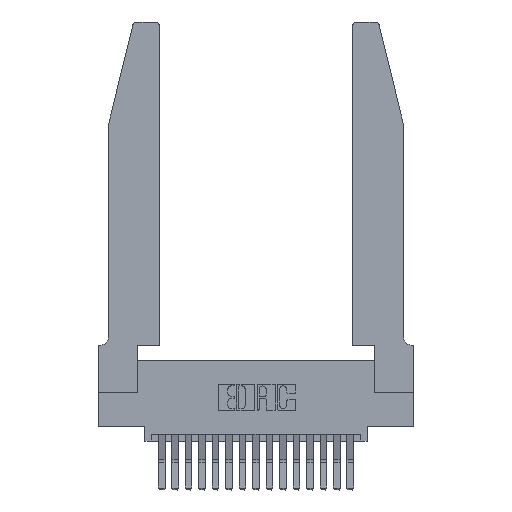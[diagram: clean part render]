
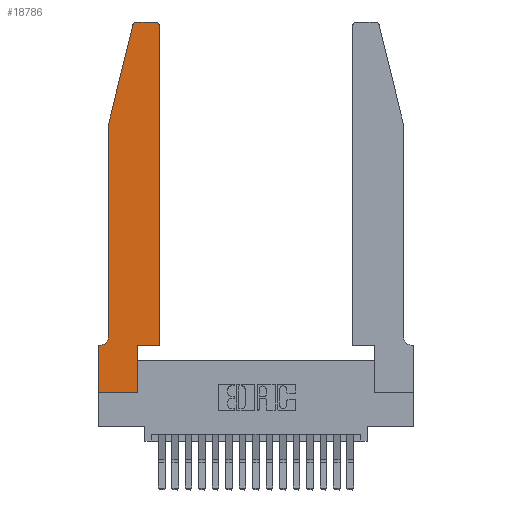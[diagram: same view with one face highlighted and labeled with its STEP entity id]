
A CAD part, top view. The second image highlights one B-rep face of the part: STEP entity #18786.
In plain terms, the highlighted planar face has unit normal (0, 0, 1).
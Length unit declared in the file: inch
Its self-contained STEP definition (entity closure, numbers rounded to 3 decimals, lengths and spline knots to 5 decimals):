
#42 = CARTESIAN_POINT ( 'NONE',  ( 0.2865, 0., 0.37 ) ) ;
#189 = DIRECTION ( 'NONE',  ( 0., -1., 0. ) ) ;
#421 = EDGE_CURVE ( 'NONE', #17162, #8743, #11018, .T. ) ;
#666 = DIRECTION ( 'NONE',  ( -1., 0., 0. ) ) ;
#910 = VERTEX_POINT ( 'NONE', #7275 ) ;
#926 = CARTESIAN_POINT ( 'NONE',  ( 0.4205, 2.75, 0.37 ) ) ;
#972 = FACE_OUTER_BOUND ( 'NONE', #2865, .T. ) ;
#1042 = ORIENTED_EDGE ( 'NONE', *, *, #15183, .T. ) ;
#1206 = VECTOR ( 'NONE', #11545, 39.37008 ) ;
#1276 = CIRCLE ( 'NONE', #7724, 0.03 ) ;
#1306 = ORIENTED_EDGE ( 'NONE', *, *, #5719, .T. ) ;
#1853 = CARTESIAN_POINT ( 'NONE',  ( 0., 0., 0.37 ) ) ;
#2221 = VECTOR ( 'NONE', #15643, 39.37008 ) ;
#2239 = CARTESIAN_POINT ( 'NONE',  ( 0.0055, 0.42, 0.37 ) ) ;
#2429 = EDGE_CURVE ( 'NONE', #5125, #6080, #3326, .T. ) ;
#2483 = CARTESIAN_POINT ( 'NONE',  ( 0., 0., 0.37 ) ) ;
#2716 = DIRECTION ( 'NONE',  ( 1., 0., 0. ) ) ;
#2790 = LINE ( 'NONE', #1853, #17548 ) ;
#2847 = VECTOR ( 'NONE', #11542, 39.37008 ) ;
#2851 = DIRECTION ( 'NONE',  ( 0., 0., 1. ) ) ;
#2865 = EDGE_LOOP ( 'NONE', ( #3240, #12995, #8635, #9447, #3397, #10828, #1042, #6276, #11467, #8108, #1306, #12363 ) ) ;
#2877 = VERTEX_POINT ( 'NONE', #7660 ) ;
#3180 = VERTEX_POINT ( 'NONE', #4149 ) ;
#3240 = ORIENTED_EDGE ( 'NONE', *, *, #4874, .T. ) ;
#3252 = AXIS2_PLACEMENT_3D ( 'NONE', #7352, #9004, #5907 ) ;
#3326 = LINE ( 'NONE', #11749, #2847 ) ;
#3397 = ORIENTED_EDGE ( 'NONE', *, *, #4354, .T. ) ;
#4139 = DIRECTION ( 'NONE',  ( -1., 0., 0. ) ) ;
#4149 = CARTESIAN_POINT ( 'NONE',  ( 0.0755, 0.42, 0.37 ) ) ;
#4354 = EDGE_CURVE ( 'NONE', #3180, #17162, #4733, .T. ) ;
#4645 = VECTOR ( 'NONE', #4139, 39.37008 ) ;
#4676 = LINE ( 'NONE', #11402, #1206 ) ;
#4733 = CIRCLE ( 'NONE', #5237, 0.07 ) ;
#4816 = AXIS2_PLACEMENT_3D ( 'NONE', #10601, #2851, #2716 ) ;
#4874 = EDGE_CURVE ( 'NONE', #13623, #910, #19231, .T. ) ;
#5013 = DIRECTION ( 'NONE',  ( 1., 0., 0. ) ) ;
#5125 = VERTEX_POINT ( 'NONE', #2483 ) ;
#5237 = AXIS2_PLACEMENT_3D ( 'NONE', #2239, #5364, #666 ) ;
#5364 = DIRECTION ( 'NONE',  ( 0., 0., -1. ) ) ;
#5719 = EDGE_CURVE ( 'NONE', #10655, #15752, #4676, .T. ) ;
#5907 = DIRECTION ( 'NONE',  ( 1., 0., 0. ) ) ;
#6080 = VERTEX_POINT ( 'NONE', #42 ) ;
#6094 = DIRECTION ( 'NONE',  ( 0., 0., 1. ) ) ;
#6276 = ORIENTED_EDGE ( 'NONE', *, *, #2429, .T. ) ;
#7275 = CARTESIAN_POINT ( 'NONE',  ( 0.284, 2.75, 0.37 ) ) ;
#7352 = CARTESIAN_POINT ( 'NONE',  ( 0., 0.35, 0.37 ) ) ;
#7660 = CARTESIAN_POINT ( 'NONE',  ( 0.0755, 2., 0.37 ) ) ;
#7667 = DIRECTION ( 'NONE',  ( 1., 0., 0. ) ) ;
#7724 = AXIS2_PLACEMENT_3D ( 'NONE', #7739, #6094, #7667 ) ;
#7739 = CARTESIAN_POINT ( 'NONE',  ( 0.4205, 2.72, 0.37 ) ) ;
#8039 = EDGE_CURVE ( 'NONE', #9073, #10655, #17857, .T. ) ;
#8108 = ORIENTED_EDGE ( 'NONE', *, *, #8039, .T. ) ;
#8635 = ORIENTED_EDGE ( 'NONE', *, *, #9545, .T. ) ;
#8743 = VERTEX_POINT ( 'NONE', #9589 ) ;
#8876 = CARTESIAN_POINT ( 'NONE',  ( 0.4505, 0.35, 0.37 ) ) ;
#9004 = DIRECTION ( 'NONE',  ( 0., 0., 1. ) ) ;
#9073 = VERTEX_POINT ( 'NONE', #12073 ) ;
#9202 = CARTESIAN_POINT ( 'NONE',  ( 0.2865, 0.35, 0.37 ) ) ;
#9447 = ORIENTED_EDGE ( 'NONE', *, *, #15302, .T. ) ;
#9545 = EDGE_CURVE ( 'NONE', #19202, #2877, #16301, .T. ) ;
#9589 = CARTESIAN_POINT ( 'NONE',  ( 0., 0.35, 0.37 ) ) ;
#9750 = DIRECTION ( 'NONE',  ( 0., -1., 0. ) ) ;
#10155 = VECTOR ( 'NONE', #9750, 39.37008 ) ;
#10344 = VECTOR ( 'NONE', #15387, 39.37008 ) ;
#10601 = CARTESIAN_POINT ( 'NONE',  ( 0.284, 2.72, 0.37 ) ) ;
#10655 = VERTEX_POINT ( 'NONE', #8876 ) ;
#10828 = ORIENTED_EDGE ( 'NONE', *, *, #421, .T. ) ;
#11018 = LINE ( 'NONE', #19846, #4645 ) ;
#11402 = CARTESIAN_POINT ( 'NONE',  ( 0.4505, 0.35, 0.37 ) ) ;
#11467 = ORIENTED_EDGE ( 'NONE', *, *, #18243, .T. ) ;
#11542 = DIRECTION ( 'NONE',  ( 1., 0., 0. ) ) ;
#11545 = DIRECTION ( 'NONE',  ( 0., 1., 0. ) ) ;
#11749 = CARTESIAN_POINT ( 'NONE',  ( 0., 0., 0.37 ) ) ;
#12073 = CARTESIAN_POINT ( 'NONE',  ( 0.2865, 0.35, 0.37 ) ) ;
#12363 = ORIENTED_EDGE ( 'NONE', *, *, #16509, .T. ) ;
#12794 = CARTESIAN_POINT ( 'NONE',  ( 0.4505, 0.35, 0.37 ) ) ;
#12995 = ORIENTED_EDGE ( 'NONE', *, *, #18398, .T. ) ;
#13339 = CARTESIAN_POINT ( 'NONE',  ( 0.0755, 2., 0.37 ) ) ;
#13466 = CARTESIAN_POINT ( 'NONE',  ( 0.4505, 2.72, 0.37 ) ) ;
#13623 = VERTEX_POINT ( 'NONE', #926 ) ;
#14281 = LINE ( 'NONE', #9202, #10344 ) ;
#14286 = CARTESIAN_POINT ( 'NONE',  ( 0.0755, 2., 0.37 ) ) ;
#14587 = CARTESIAN_POINT ( 'NONE',  ( 0.0055, 0.35, 0.37 ) ) ;
#14682 = CARTESIAN_POINT ( 'NONE',  ( 0.25487, 2.72718, 0.37 ) ) ;
#15183 = EDGE_CURVE ( 'NONE', #8743, #5125, #2790, .T. ) ;
#15302 = EDGE_CURVE ( 'NONE', #2877, #3180, #18551, .T. ) ;
#15387 = DIRECTION ( 'NONE',  ( 0., 1., 0. ) ) ;
#15643 = DIRECTION ( 'NONE',  ( -1., 0., 0. ) ) ;
#15752 = VERTEX_POINT ( 'NONE', #13466 ) ;
#15770 = CARTESIAN_POINT ( 'NONE',  ( 0.2605, 2.75, 0.37 ) ) ;
#16301 = LINE ( 'NONE', #13339, #20246 ) ;
#16509 = EDGE_CURVE ( 'NONE', #15752, #13623, #1276, .T. ) ;
#17162 = VERTEX_POINT ( 'NONE', #14587 ) ;
#17548 = VECTOR ( 'NONE', #189, 39.37008 ) ;
#17857 = LINE ( 'NONE', #12794, #19095 ) ;
#18243 = EDGE_CURVE ( 'NONE', #6080, #9073, #14281, .T. ) ;
#18247 = DIRECTION ( 'NONE',  ( -0.239, -0.971, 0. ) ) ;
#18398 = EDGE_CURVE ( 'NONE', #910, #19202, #19732, .T. ) ;
#18433 = PLANE ( 'NONE',  #3252 ) ;
#18551 = LINE ( 'NONE', #14286, #10155 ) ;
#18786 = ADVANCED_FACE ( 'NONE', ( #972 ), #18433, .T. ) ;
#19095 = VECTOR ( 'NONE', #5013, 39.37008 ) ;
#19202 = VERTEX_POINT ( 'NONE', #14682 ) ;
#19231 = LINE ( 'NONE', #15770, #2221 ) ;
#19732 = CIRCLE ( 'NONE', #4816, 0.03 ) ;
#19846 = CARTESIAN_POINT ( 'NONE',  ( 0.0755, 0.35, 0.37 ) ) ;
#20246 = VECTOR ( 'NONE', #18247, 39.37008 ) ;
